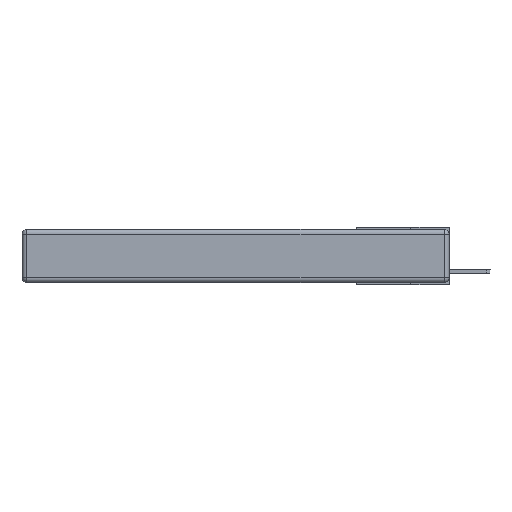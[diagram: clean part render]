
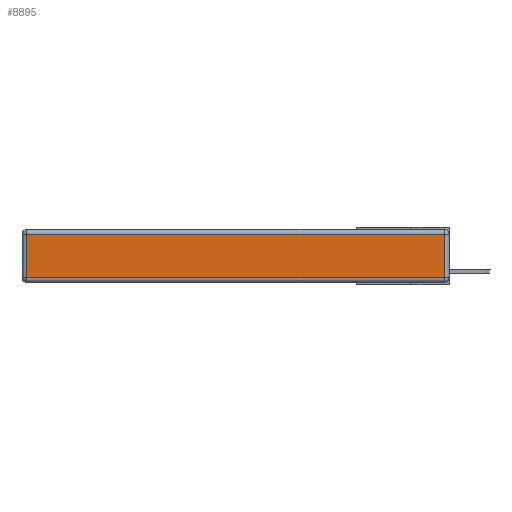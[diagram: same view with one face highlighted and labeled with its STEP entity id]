
A CAD part, left-side view. The second image highlights one B-rep face of the part: STEP entity #8895.
In plain terms, the highlighted planar face has unit normal (-1, 0, 0).
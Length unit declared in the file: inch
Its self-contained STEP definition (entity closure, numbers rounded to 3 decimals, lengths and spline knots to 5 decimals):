
#770 = VERTEX_POINT ( 'NONE', #3504 ) ;
#902 = ORIENTED_EDGE ( 'NONE', *, *, #11638, .T. ) ;
#1054 = ORIENTED_EDGE ( 'NONE', *, *, #7546, .T. ) ;
#3042 = DIRECTION ( 'NONE',  ( 0., -1., 0. ) ) ;
#3504 = CARTESIAN_POINT ( 'NONE',  ( 0., 0.03, -0.313 ) ) ;
#3543 = LINE ( 'NONE', #8163, #9275 ) ;
#3850 = AXIS2_PLACEMENT_3D ( 'NONE', #5232, #11946, #6208 ) ;
#4082 = VERTEX_POINT ( 'NONE', #7273 ) ;
#4109 = DIRECTION ( 'NONE',  ( 0., 0., -1. ) ) ;
#5171 = VERTEX_POINT ( 'NONE', #9373 ) ;
#5232 = CARTESIAN_POINT ( 'NONE',  ( 0., 0., -0.343 ) ) ;
#5340 = VERTEX_POINT ( 'NONE', #5886 ) ;
#5680 = EDGE_CURVE ( 'NONE', #770, #5171, #6368, .T. ) ;
#5863 = ORIENTED_EDGE ( 'NONE', *, *, #5680, .T. ) ;
#5886 = CARTESIAN_POINT ( 'NONE',  ( 0., 2.72, -0.313 ) ) ;
#6208 = DIRECTION ( 'NONE',  ( 0., 0., 1. ) ) ;
#6368 = LINE ( 'NONE', #11958, #9813 ) ;
#6890 = VECTOR ( 'NONE', #4109, 39.37008 ) ;
#7237 = DIRECTION ( 'NONE',  ( 0., 0., 1. ) ) ;
#7273 = CARTESIAN_POINT ( 'NONE',  ( 0., 2.72, -0.03 ) ) ;
#7546 = EDGE_CURVE ( 'NONE', #5340, #770, #12286, .T. ) ;
#7635 = LINE ( 'NONE', #11767, #6890 ) ;
#8163 = CARTESIAN_POINT ( 'NONE',  ( 0., 2.75, -0.03 ) ) ;
#8371 = EDGE_LOOP ( 'NONE', ( #1054, #5863, #902, #10148 ) ) ;
#8527 = EDGE_CURVE ( 'NONE', #4082, #5340, #7635, .T. ) ;
#8688 = FACE_OUTER_BOUND ( 'NONE', #8371, .T. ) ;
#8895 = ADVANCED_FACE ( 'NONE', ( #8688 ), #9063, .T. ) ;
#9063 = PLANE ( 'NONE',  #3850 ) ;
#9088 = DIRECTION ( 'NONE',  ( 0., 1., 0. ) ) ;
#9275 = VECTOR ( 'NONE', #9088, 39.37008 ) ;
#9314 = VECTOR ( 'NONE', #3042, 39.37008 ) ;
#9373 = CARTESIAN_POINT ( 'NONE',  ( 0., 0.03, -0.03 ) ) ;
#9813 = VECTOR ( 'NONE', #7237, 39.37008 ) ;
#10148 = ORIENTED_EDGE ( 'NONE', *, *, #8527, .T. ) ;
#11604 = CARTESIAN_POINT ( 'NONE',  ( 0., 0., -0.313 ) ) ;
#11638 = EDGE_CURVE ( 'NONE', #5171, #4082, #3543, .T. ) ;
#11767 = CARTESIAN_POINT ( 'NONE',  ( 0., 2.72, -0.343 ) ) ;
#11946 = DIRECTION ( 'NONE',  ( -1., 0., 0. ) ) ;
#11958 = CARTESIAN_POINT ( 'NONE',  ( 0., 0.03, -0.343 ) ) ;
#12286 = LINE ( 'NONE', #11604, #9314 ) ;
